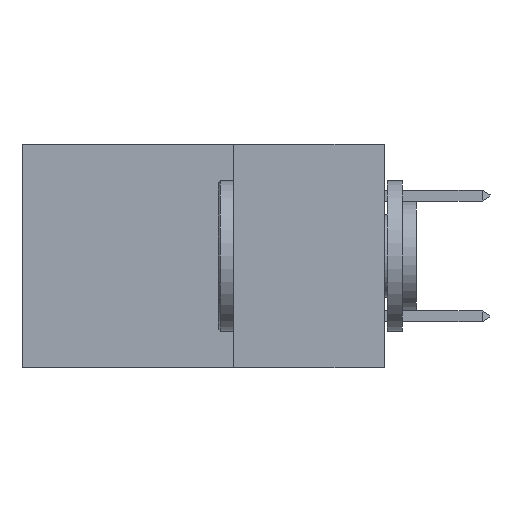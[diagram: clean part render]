
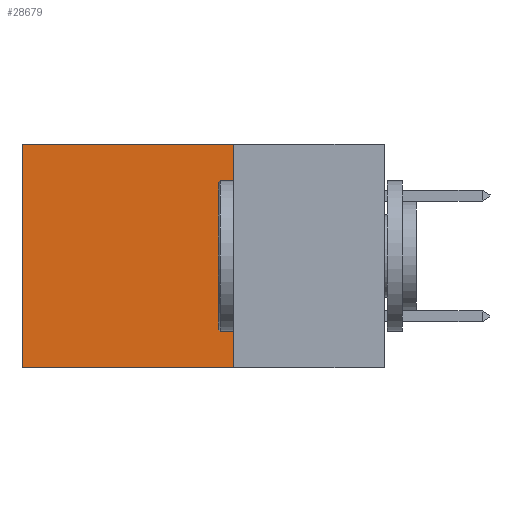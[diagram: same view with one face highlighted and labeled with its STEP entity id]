
A CAD part, left-side view. The second image highlights one B-rep face of the part: STEP entity #28679.
In plain terms, the highlighted planar face has unit normal (-1, 0, 0).
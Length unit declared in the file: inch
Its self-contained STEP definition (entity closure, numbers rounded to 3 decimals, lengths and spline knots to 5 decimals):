
#1403 = CARTESIAN_POINT ( 'NONE',  ( 0.2875, 0.25, 0. ) ) ;
#3528 = LINE ( 'NONE', #8723, #27768 ) ;
#4415 = CARTESIAN_POINT ( 'NONE',  ( 0.2875, 0.6, -0.37 ) ) ;
#4779 = CARTESIAN_POINT ( 'NONE',  ( 0.2875, 0.25, 0. ) ) ;
#4815 = VERTEX_POINT ( 'NONE', #21242 ) ;
#4918 = PLANE ( 'NONE',  #6789 ) ;
#5526 = DIRECTION ( 'NONE',  ( 0., 1., 0. ) ) ;
#5734 = CARTESIAN_POINT ( 'NONE',  ( 0.2875, 0.25, -0.37 ) ) ;
#6789 = AXIS2_PLACEMENT_3D ( 'NONE', #4779, #26999, #8109 ) ;
#7553 = VECTOR ( 'NONE', #12109, 39.37008 ) ;
#8075 = CARTESIAN_POINT ( 'NONE',  ( 0.2875, 0.6, 0. ) ) ;
#8109 = DIRECTION ( 'NONE',  ( 0., 0., -1. ) ) ;
#8723 = CARTESIAN_POINT ( 'NONE',  ( 0.2875, 0.25, 0. ) ) ;
#9878 = FACE_OUTER_BOUND ( 'NONE', #40290, .T. ) ;
#11050 = ORIENTED_EDGE ( 'NONE', *, *, #12236, .T. ) ;
#11241 = DIRECTION ( 'NONE',  ( 0., 0., -1. ) ) ;
#11981 = CARTESIAN_POINT ( 'NONE',  ( 0.2875, 0.25, -0.37 ) ) ;
#12109 = DIRECTION ( 'NONE',  ( 0., 1., 0. ) ) ;
#12236 = EDGE_CURVE ( 'NONE', #19176, #4815, #3528, .T. ) ;
#12326 = ORIENTED_EDGE ( 'NONE', *, *, #37388, .F. ) ;
#12962 = VERTEX_POINT ( 'NONE', #11981 ) ;
#14259 = LINE ( 'NONE', #17347, #38395 ) ;
#14284 = DIRECTION ( 'NONE',  ( 0., 0., -1. ) ) ;
#17347 = CARTESIAN_POINT ( 'NONE',  ( 0.2875, 0.25, 0. ) ) ;
#18425 = VERTEX_POINT ( 'NONE', #4415 ) ;
#19176 = VERTEX_POINT ( 'NONE', #1403 ) ;
#19813 = LINE ( 'NONE', #8075, #35576 ) ;
#21242 = CARTESIAN_POINT ( 'NONE',  ( 0.2875, 0.6, 0. ) ) ;
#26999 = DIRECTION ( 'NONE',  ( 1., 0., 0. ) ) ;
#27335 = EDGE_CURVE ( 'NONE', #4815, #18425, #19813, .T. ) ;
#27768 = VECTOR ( 'NONE', #5526, 39.37008 ) ;
#28028 = ORIENTED_EDGE ( 'NONE', *, *, #27335, .T. ) ;
#28679 = ADVANCED_FACE ( 'NONE', ( #9878 ), #4918, .F. ) ;
#29257 = EDGE_CURVE ( 'NONE', #19176, #12962, #14259, .T. ) ;
#35576 = VECTOR ( 'NONE', #11241, 39.37008 ) ;
#37388 = EDGE_CURVE ( 'NONE', #12962, #18425, #40106, .T. ) ;
#38395 = VECTOR ( 'NONE', #14284, 39.37008 ) ;
#38612 = ORIENTED_EDGE ( 'NONE', *, *, #29257, .F. ) ;
#40106 = LINE ( 'NONE', #5734, #7553 ) ;
#40290 = EDGE_LOOP ( 'NONE', ( #28028, #12326, #38612, #11050 ) ) ;
